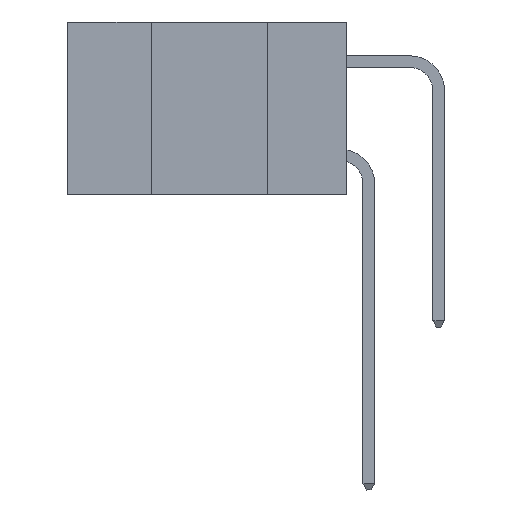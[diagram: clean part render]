
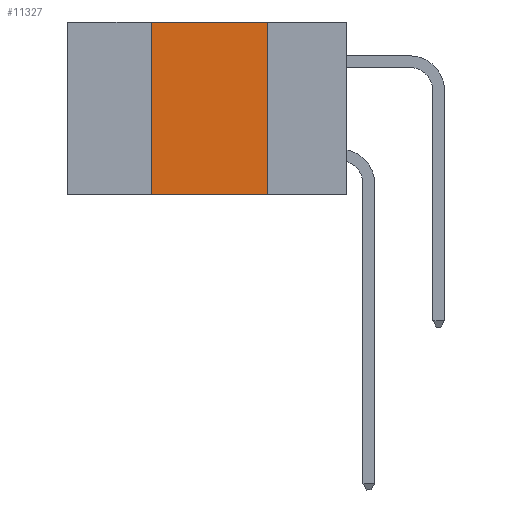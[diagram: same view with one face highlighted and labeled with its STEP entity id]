
A CAD part, left-side view. The second image highlights one B-rep face of the part: STEP entity #11327.
In plain terms, the highlighted planar face has unit normal (-1, 0, 0).
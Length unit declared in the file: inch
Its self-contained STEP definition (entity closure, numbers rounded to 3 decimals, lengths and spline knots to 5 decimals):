
#1043 = VERTEX_POINT ( 'NONE', #6068 ) ;
#1817 = VERTEX_POINT ( 'NONE', #8287 ) ;
#2359 = DIRECTION ( 'NONE',  ( 0., 0., -1. ) ) ;
#2755 = VECTOR ( 'NONE', #18194, 39.37008 ) ;
#4011 = PLANE ( 'NONE',  #10135 ) ;
#4044 = CARTESIAN_POINT ( 'NONE',  ( 0., 0.17, 0. ) ) ;
#5744 = DIRECTION ( 'NONE',  ( 0., 0., -1. ) ) ;
#5802 = LINE ( 'NONE', #20648, #10217 ) ;
#6068 = CARTESIAN_POINT ( 'NONE',  ( 0., 0.17, -0.37 ) ) ;
#6454 = VERTEX_POINT ( 'NONE', #12236 ) ;
#6529 = CARTESIAN_POINT ( 'NONE',  ( 0., 0.6, -0.37 ) ) ;
#6729 = LINE ( 'NONE', #6529, #2755 ) ;
#8036 = VECTOR ( 'NONE', #5744, 39.37008 ) ;
#8245 = FACE_OUTER_BOUND ( 'NONE', #12104, .T. ) ;
#8287 = CARTESIAN_POINT ( 'NONE',  ( 0., 0.17, 0. ) ) ;
#8431 = VERTEX_POINT ( 'NONE', #20902 ) ;
#8829 = ORIENTED_EDGE ( 'NONE', *, *, #20913, .F. ) ;
#9364 = ORIENTED_EDGE ( 'NONE', *, *, #19881, .T. ) ;
#9559 = VECTOR ( 'NONE', #21071, 39.37008 ) ;
#10135 = AXIS2_PLACEMENT_3D ( 'NONE', #19066, #12417, #2359 ) ;
#10217 = VECTOR ( 'NONE', #10665, 39.37008 ) ;
#10665 = DIRECTION ( 'NONE',  ( 0., -1., 0. ) ) ;
#11327 = ADVANCED_FACE ( 'NONE', ( #8245 ), #4011, .F. ) ;
#11454 = EDGE_CURVE ( 'NONE', #8431, #6454, #19492, .T. ) ;
#12104 = EDGE_LOOP ( 'NONE', ( #17182, #8829, #13264, #9364 ) ) ;
#12236 = CARTESIAN_POINT ( 'NONE',  ( 0., 0.42, 0. ) ) ;
#12417 = DIRECTION ( 'NONE',  ( 1., 0., 0. ) ) ;
#13264 = ORIENTED_EDGE ( 'NONE', *, *, #11454, .F. ) ;
#17182 = ORIENTED_EDGE ( 'NONE', *, *, #19606, .F. ) ;
#17442 = LINE ( 'NONE', #4044, #8036 ) ;
#17737 = CARTESIAN_POINT ( 'NONE',  ( 0., 0.42, 0. ) ) ;
#18194 = DIRECTION ( 'NONE',  ( 0., -1., 0. ) ) ;
#19066 = CARTESIAN_POINT ( 'NONE',  ( 0., 0.6, 0. ) ) ;
#19492 = LINE ( 'NONE', #17737, #9559 ) ;
#19606 = EDGE_CURVE ( 'NONE', #1817, #1043, #17442, .T. ) ;
#19881 = EDGE_CURVE ( 'NONE', #8431, #1043, #6729, .T. ) ;
#20648 = CARTESIAN_POINT ( 'NONE',  ( 0., 0.6, 0. ) ) ;
#20902 = CARTESIAN_POINT ( 'NONE',  ( 0., 0.42, -0.37 ) ) ;
#20913 = EDGE_CURVE ( 'NONE', #6454, #1817, #5802, .T. ) ;
#21071 = DIRECTION ( 'NONE',  ( 0., 0., 1. ) ) ;
